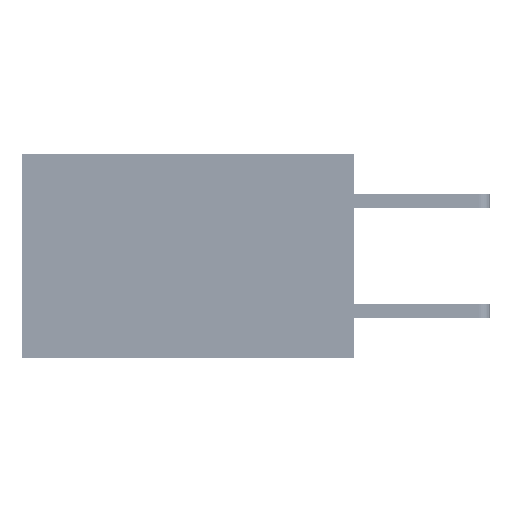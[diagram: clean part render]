
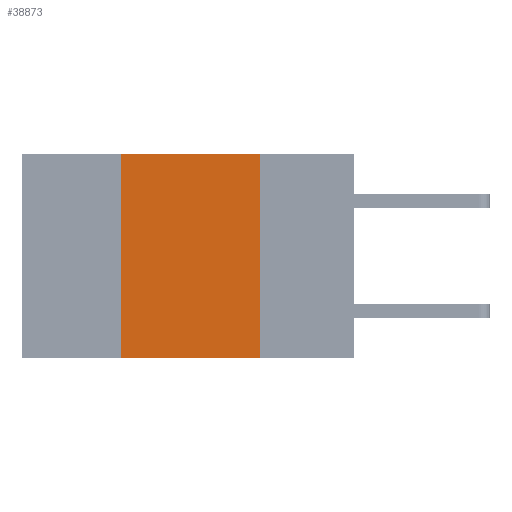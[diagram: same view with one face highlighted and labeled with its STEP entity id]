
A CAD part, left-side view. The second image highlights one B-rep face of the part: STEP entity #38873.
In plain terms, the highlighted planar face has unit normal (-1, 0, 0).
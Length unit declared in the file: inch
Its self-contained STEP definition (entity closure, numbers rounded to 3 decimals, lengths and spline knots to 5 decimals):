
#318 = ORIENTED_EDGE ( 'NONE', *, *, #10252, .T. ) ;
#2808 = DIRECTION ( 'NONE',  ( 0., 0., -1. ) ) ;
#5250 = LINE ( 'NONE', #25687, #28886 ) ;
#5826 = CARTESIAN_POINT ( 'NONE',  ( 0., 0.6, 0. ) ) ;
#7163 = LINE ( 'NONE', #35549, #34557 ) ;
#8135 = VERTEX_POINT ( 'NONE', #21606 ) ;
#10252 = EDGE_CURVE ( 'NONE', #45822, #13985, #7163, .T. ) ;
#12090 = ORIENTED_EDGE ( 'NONE', *, *, #40411, .F. ) ;
#13985 = VERTEX_POINT ( 'NONE', #29694 ) ;
#14112 = AXIS2_PLACEMENT_3D ( 'NONE', #30945, #39152, #2808 ) ;
#18503 = FACE_OUTER_BOUND ( 'NONE', #42497, .T. ) ;
#18760 = PLANE ( 'NONE',  #14112 ) ;
#21033 = VERTEX_POINT ( 'NONE', #45430 ) ;
#21606 = CARTESIAN_POINT ( 'NONE',  ( 0., 0.42, 0. ) ) ;
#22367 = VECTOR ( 'NONE', #22796, 39.37008 ) ;
#22796 = DIRECTION ( 'NONE',  ( 0., -1., 0. ) ) ;
#25687 = CARTESIAN_POINT ( 'NONE',  ( 0., 0.17, 0. ) ) ;
#27763 = LINE ( 'NONE', #43945, #44332 ) ;
#28886 = VECTOR ( 'NONE', #45365, 39.37008 ) ;
#29596 = DIRECTION ( 'NONE',  ( 0., 0., 1. ) ) ;
#29694 = CARTESIAN_POINT ( 'NONE',  ( 0., 0.17, -0.37 ) ) ;
#29794 = EDGE_CURVE ( 'NONE', #21033, #13985, #5250, .T. ) ;
#30945 = CARTESIAN_POINT ( 'NONE',  ( 0., 0.6, 0. ) ) ;
#34271 = EDGE_CURVE ( 'NONE', #8135, #21033, #42189, .T. ) ;
#34557 = VECTOR ( 'NONE', #51244, 39.37008 ) ;
#35549 = CARTESIAN_POINT ( 'NONE',  ( 0., 0.6, -0.37 ) ) ;
#36311 = ORIENTED_EDGE ( 'NONE', *, *, #29794, .F. ) ;
#38873 = ADVANCED_FACE ( 'NONE', ( #18503 ), #18760, .F. ) ;
#39152 = DIRECTION ( 'NONE',  ( 1., 0., 0. ) ) ;
#39469 = CARTESIAN_POINT ( 'NONE',  ( 0., 0.42, -0.37 ) ) ;
#40411 = EDGE_CURVE ( 'NONE', #45822, #8135, #27763, .T. ) ;
#42189 = LINE ( 'NONE', #5826, #22367 ) ;
#42497 = EDGE_LOOP ( 'NONE', ( #36311, #49888, #12090, #318 ) ) ;
#43945 = CARTESIAN_POINT ( 'NONE',  ( 0., 0.42, 0. ) ) ;
#44332 = VECTOR ( 'NONE', #29596, 39.37008 ) ;
#45365 = DIRECTION ( 'NONE',  ( 0., 0., -1. ) ) ;
#45430 = CARTESIAN_POINT ( 'NONE',  ( 0., 0.17, 0. ) ) ;
#45822 = VERTEX_POINT ( 'NONE', #39469 ) ;
#49888 = ORIENTED_EDGE ( 'NONE', *, *, #34271, .F. ) ;
#51244 = DIRECTION ( 'NONE',  ( 0., -1., 0. ) ) ;
